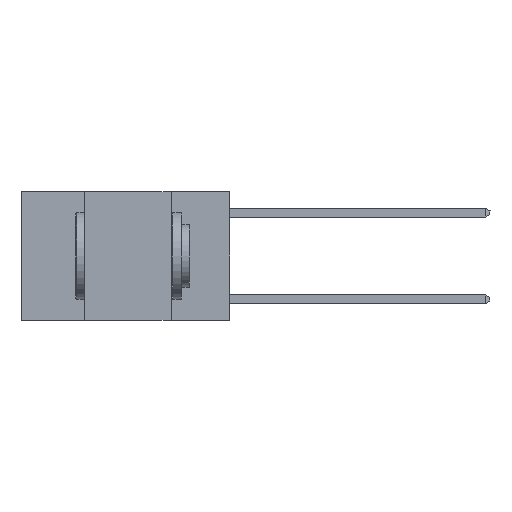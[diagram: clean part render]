
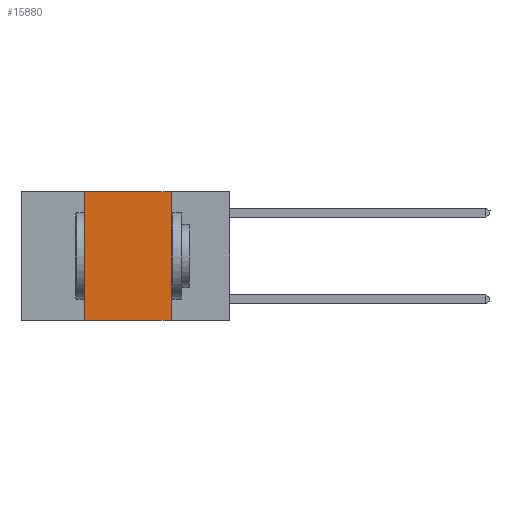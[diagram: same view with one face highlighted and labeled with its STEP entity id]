
A CAD part, left-side view. The second image highlights one B-rep face of the part: STEP entity #15880.
In plain terms, the highlighted planar face has unit normal (-1, 0, 0).
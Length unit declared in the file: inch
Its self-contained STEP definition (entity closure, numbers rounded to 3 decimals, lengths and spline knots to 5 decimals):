
#439 = LINE ( 'NONE', #3402, #4997 ) ;
#740 = LINE ( 'NONE', #3501, #5649 ) ;
#746 = LINE ( 'NONE', #18662, #18067 ) ;
#1077 = ORIENTED_EDGE ( 'NONE', *, *, #10827, .F. ) ;
#1273 = VERTEX_POINT ( 'NONE', #16914 ) ;
#1292 = EDGE_CURVE ( 'NONE', #6801, #1273, #740, .T. ) ;
#2647 = AXIS2_PLACEMENT_3D ( 'NONE', #8522, #8625, #19186 ) ;
#2764 = FACE_OUTER_BOUND ( 'NONE', #10502, .T. ) ;
#3402 = CARTESIAN_POINT ( 'NONE',  ( 0., 0.6, -0.37 ) ) ;
#3452 = EDGE_CURVE ( 'NONE', #1273, #3835, #746, .T. ) ;
#3501 = CARTESIAN_POINT ( 'NONE',  ( 0., 0.42, 0. ) ) ;
#3571 = CARTESIAN_POINT ( 'NONE',  ( 0., 0.17, 0. ) ) ;
#3835 = VERTEX_POINT ( 'NONE', #9643 ) ;
#4997 = VECTOR ( 'NONE', #12195, 39.37008 ) ;
#5263 = DIRECTION ( 'NONE',  ( 0., -1., 0. ) ) ;
#5649 = VECTOR ( 'NONE', #9462, 39.37008 ) ;
#6801 = VERTEX_POINT ( 'NONE', #14439 ) ;
#6881 = PLANE ( 'NONE',  #2647 ) ;
#7200 = CARTESIAN_POINT ( 'NONE',  ( 0., 0.17, -0.37 ) ) ;
#8522 = CARTESIAN_POINT ( 'NONE',  ( 0., 0.6, 0. ) ) ;
#8625 = DIRECTION ( 'NONE',  ( 1., 0., 0. ) ) ;
#8642 = VERTEX_POINT ( 'NONE', #7200 ) ;
#9091 = LINE ( 'NONE', #3571, #17204 ) ;
#9462 = DIRECTION ( 'NONE',  ( 0., 0., 1. ) ) ;
#9643 = CARTESIAN_POINT ( 'NONE',  ( 0., 0.17, 0. ) ) ;
#9694 = EDGE_CURVE ( 'NONE', #6801, #8642, #439, .T. ) ;
#10045 = ORIENTED_EDGE ( 'NONE', *, *, #9694, .T. ) ;
#10502 = EDGE_LOOP ( 'NONE', ( #1077, #17133, #14166, #10045 ) ) ;
#10827 = EDGE_CURVE ( 'NONE', #3835, #8642, #9091, .T. ) ;
#11089 = DIRECTION ( 'NONE',  ( 0., 0., -1. ) ) ;
#12195 = DIRECTION ( 'NONE',  ( 0., -1., 0. ) ) ;
#14166 = ORIENTED_EDGE ( 'NONE', *, *, #1292, .F. ) ;
#14439 = CARTESIAN_POINT ( 'NONE',  ( 0., 0.42, -0.37 ) ) ;
#15880 = ADVANCED_FACE ( 'NONE', ( #2764 ), #6881, .F. ) ;
#16914 = CARTESIAN_POINT ( 'NONE',  ( 0., 0.42, 0. ) ) ;
#17133 = ORIENTED_EDGE ( 'NONE', *, *, #3452, .F. ) ;
#17204 = VECTOR ( 'NONE', #11089, 39.37008 ) ;
#18067 = VECTOR ( 'NONE', #5263, 39.37008 ) ;
#18662 = CARTESIAN_POINT ( 'NONE',  ( 0., 0.6, 0. ) ) ;
#19186 = DIRECTION ( 'NONE',  ( 0., 0., -1. ) ) ;
